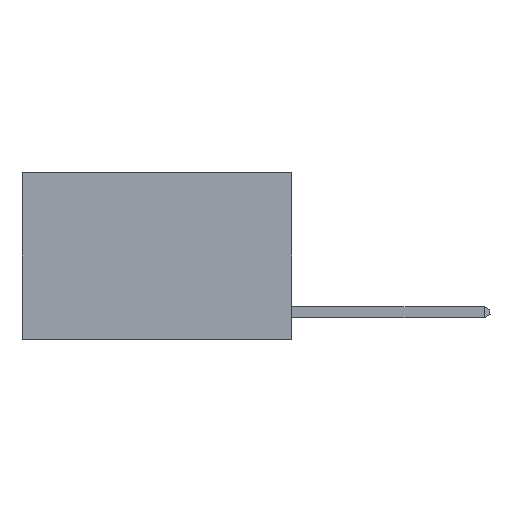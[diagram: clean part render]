
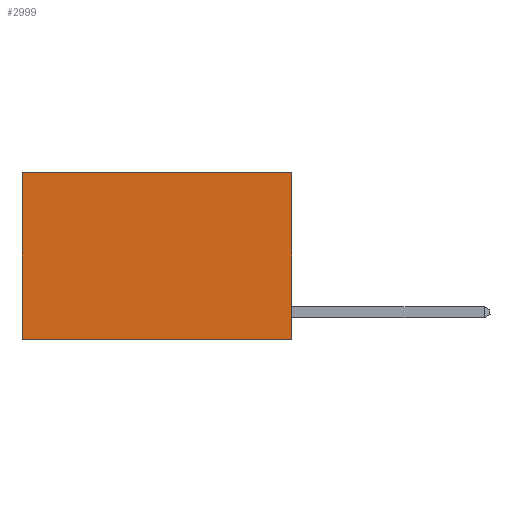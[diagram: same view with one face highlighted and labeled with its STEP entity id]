
A CAD part, left-side view. The second image highlights one B-rep face of the part: STEP entity #2999.
In plain terms, the highlighted planar face has unit normal (-1, 0, 0).
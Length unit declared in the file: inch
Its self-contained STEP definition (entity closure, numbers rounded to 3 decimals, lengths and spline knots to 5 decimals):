
#205 = ORIENTED_EDGE ( 'NONE', *, *, #6921, .T. ) ;
#685 = VERTEX_POINT ( 'NONE', #6961 ) ;
#1059 = ORIENTED_EDGE ( 'NONE', *, *, #7584, .F. ) ;
#1176 = ORIENTED_EDGE ( 'NONE', *, *, #6659, .F. ) ;
#1188 = VECTOR ( 'NONE', #7665, 39.37008 ) ;
#1266 = VERTEX_POINT ( 'NONE', #4438 ) ;
#1275 = ORIENTED_EDGE ( 'NONE', *, *, #2173, .T. ) ;
#2173 = EDGE_CURVE ( 'NONE', #685, #1266, #7797, .T. ) ;
#2999 = ADVANCED_FACE ( 'NONE', ( #6096 ), #6297, .F. ) ;
#3078 = EDGE_LOOP ( 'NONE', ( #205, #1059, #1176, #1275 ) ) ;
#3429 = DIRECTION ( 'NONE',  ( 0., 1., 0. ) ) ;
#3450 = VECTOR ( 'NONE', #3550, 39.37008 ) ;
#3550 = DIRECTION ( 'NONE',  ( 0., 0., -1. ) ) ;
#3704 = VERTEX_POINT ( 'NONE', #6119 ) ;
#3953 = CARTESIAN_POINT ( 'NONE',  ( 0.2625, 0.6, 0. ) ) ;
#3965 = CARTESIAN_POINT ( 'NONE',  ( 0.2625, 0., 0. ) ) ;
#4366 = LINE ( 'NONE', #3965, #6287 ) ;
#4438 = CARTESIAN_POINT ( 'NONE',  ( 0.2625, 0.6, 0. ) ) ;
#5487 = VERTEX_POINT ( 'NONE', #8227 ) ;
#6096 = FACE_OUTER_BOUND ( 'NONE', #3078, .T. ) ;
#6119 = CARTESIAN_POINT ( 'NONE',  ( 0.2625, 0.6, -0.37 ) ) ;
#6248 = LINE ( 'NONE', #7695, #1188 ) ;
#6287 = VECTOR ( 'NONE', #10138, 39.37008 ) ;
#6297 = PLANE ( 'NONE',  #7007 ) ;
#6353 = DIRECTION ( 'NONE',  ( 0., 0., -1. ) ) ;
#6659 = EDGE_CURVE ( 'NONE', #685, #5487, #4366, .T. ) ;
#6845 = DIRECTION ( 'NONE',  ( 1., 0., 0. ) ) ;
#6921 = EDGE_CURVE ( 'NONE', #1266, #3704, #9611, .T. ) ;
#6961 = CARTESIAN_POINT ( 'NONE',  ( 0.2625, 0., 0. ) ) ;
#7007 = AXIS2_PLACEMENT_3D ( 'NONE', #10139, #6845, #6353 ) ;
#7584 = EDGE_CURVE ( 'NONE', #5487, #3704, #6248, .T. ) ;
#7665 = DIRECTION ( 'NONE',  ( 0., 1., 0. ) ) ;
#7695 = CARTESIAN_POINT ( 'NONE',  ( 0.2625, 0., -0.37 ) ) ;
#7797 = LINE ( 'NONE', #9762, #7823 ) ;
#7823 = VECTOR ( 'NONE', #3429, 39.37008 ) ;
#8227 = CARTESIAN_POINT ( 'NONE',  ( 0.2625, 0., -0.37 ) ) ;
#9611 = LINE ( 'NONE', #3953, #3450 ) ;
#9762 = CARTESIAN_POINT ( 'NONE',  ( 0.2625, 0., 0. ) ) ;
#10138 = DIRECTION ( 'NONE',  ( 0., 0., -1. ) ) ;
#10139 = CARTESIAN_POINT ( 'NONE',  ( 0.2625, 0., 0. ) ) ;
